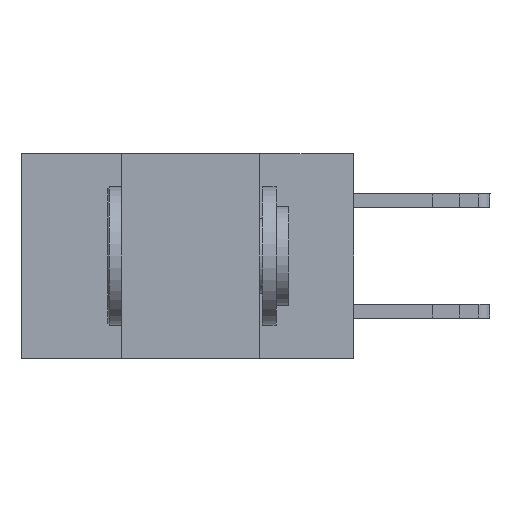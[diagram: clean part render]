
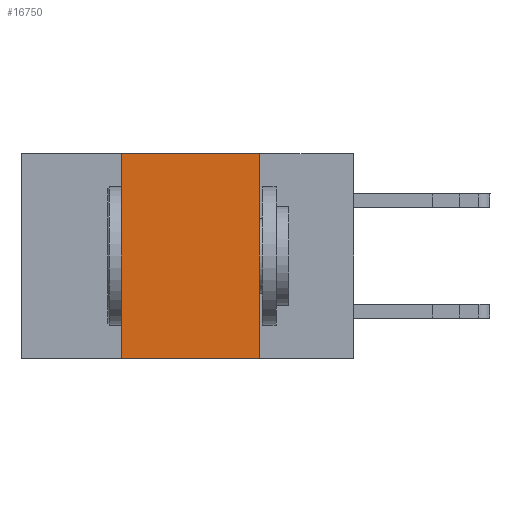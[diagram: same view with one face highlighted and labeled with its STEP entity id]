
A CAD part, left-side view. The second image highlights one B-rep face of the part: STEP entity #16750.
In plain terms, the highlighted planar face has unit normal (-1, 0, 0).
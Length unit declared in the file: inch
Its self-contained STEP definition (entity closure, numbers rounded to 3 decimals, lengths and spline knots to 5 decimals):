
#82 = CARTESIAN_POINT ( 'NONE',  ( 0., 0.42, 0. ) ) ;
#162 = DIRECTION ( 'NONE',  ( 0., 0., -1. ) ) ;
#588 = DIRECTION ( 'NONE',  ( 1., 0., 0. ) ) ;
#2282 = DIRECTION ( 'NONE',  ( 0., -1., 0. ) ) ;
#3757 = DIRECTION ( 'NONE',  ( 0., 0., -1. ) ) ;
#4059 = CARTESIAN_POINT ( 'NONE',  ( 0., 0.6, -0.37 ) ) ;
#4977 = LINE ( 'NONE', #4059, #32373 ) ;
#5028 = PLANE ( 'NONE',  #33427 ) ;
#5749 = VECTOR ( 'NONE', #2282, 39.37008 ) ;
#6077 = CARTESIAN_POINT ( 'NONE',  ( 0., 0.6, 0. ) ) ;
#8388 = EDGE_CURVE ( 'NONE', #32267, #26337, #4977, .T. ) ;
#8746 = EDGE_CURVE ( 'NONE', #32982, #21736, #12836, .T. ) ;
#10779 = LINE ( 'NONE', #16549, #21220 ) ;
#12126 = ORIENTED_EDGE ( 'NONE', *, *, #8746, .F. ) ;
#12836 = LINE ( 'NONE', #6077, #5749 ) ;
#13208 = FACE_OUTER_BOUND ( 'NONE', #30086, .T. ) ;
#13298 = DIRECTION ( 'NONE',  ( 0., 0., 1. ) ) ;
#14165 = EDGE_CURVE ( 'NONE', #21736, #26337, #10779, .T. ) ;
#16549 = CARTESIAN_POINT ( 'NONE',  ( 0., 0.17, 0. ) ) ;
#16750 = ADVANCED_FACE ( 'NONE', ( #13208 ), #5028, .F. ) ;
#17494 = ORIENTED_EDGE ( 'NONE', *, *, #30417, .F. ) ;
#18345 = VECTOR ( 'NONE', #13298, 39.37008 ) ;
#20439 = CARTESIAN_POINT ( 'NONE',  ( 0., 0.17, -0.37 ) ) ;
#21066 = CARTESIAN_POINT ( 'NONE',  ( 0., 0.6, 0. ) ) ;
#21220 = VECTOR ( 'NONE', #3757, 39.37008 ) ;
#21736 = VERTEX_POINT ( 'NONE', #33987 ) ;
#24353 = CARTESIAN_POINT ( 'NONE',  ( 0., 0.42, -0.37 ) ) ;
#26337 = VERTEX_POINT ( 'NONE', #20439 ) ;
#27616 = DIRECTION ( 'NONE',  ( 0., -1., 0. ) ) ;
#28515 = ORIENTED_EDGE ( 'NONE', *, *, #14165, .F. ) ;
#29573 = LINE ( 'NONE', #82, #18345 ) ;
#29883 = ORIENTED_EDGE ( 'NONE', *, *, #8388, .T. ) ;
#30086 = EDGE_LOOP ( 'NONE', ( #28515, #12126, #17494, #29883 ) ) ;
#30417 = EDGE_CURVE ( 'NONE', #32267, #32982, #29573, .T. ) ;
#32267 = VERTEX_POINT ( 'NONE', #24353 ) ;
#32373 = VECTOR ( 'NONE', #27616, 39.37008 ) ;
#32642 = CARTESIAN_POINT ( 'NONE',  ( 0., 0.42, 0. ) ) ;
#32982 = VERTEX_POINT ( 'NONE', #32642 ) ;
#33427 = AXIS2_PLACEMENT_3D ( 'NONE', #21066, #588, #162 ) ;
#33987 = CARTESIAN_POINT ( 'NONE',  ( 0., 0.17, 0. ) ) ;
